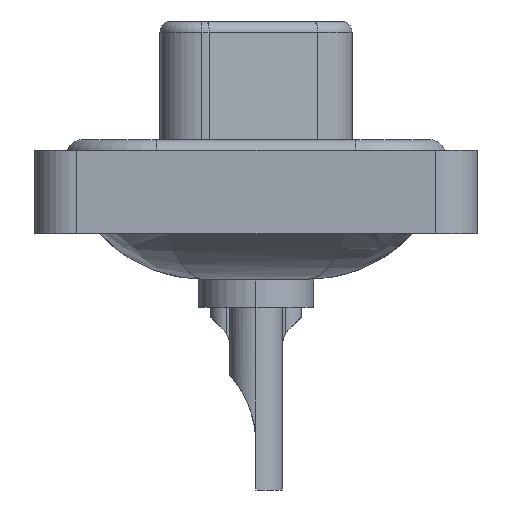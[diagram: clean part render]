
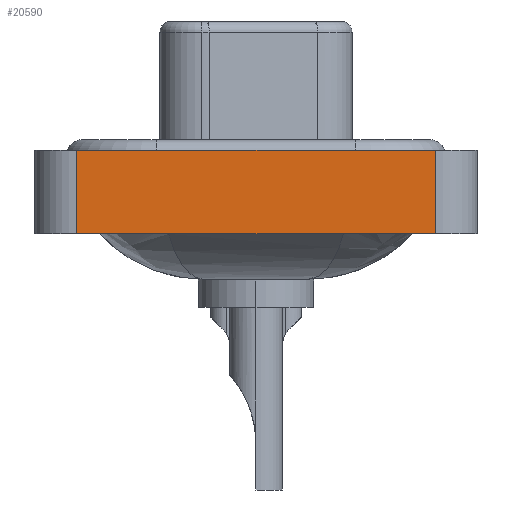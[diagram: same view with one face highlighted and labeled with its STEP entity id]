
A CAD part, left-side view. The second image highlights one B-rep face of the part: STEP entity #20590.
In plain terms, the highlighted planar face has unit normal (-1, 0, 0).
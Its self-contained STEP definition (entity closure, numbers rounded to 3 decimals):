
#236 = ORIENTED_EDGE ( 'NONE', *, *, #13467, .F. ) ;
#2484 = DIRECTION ( 'NONE',  ( 0., 0., 1. ) ) ;
#3083 = FACE_OUTER_BOUND ( 'NONE', #12416, .T. ) ;
#3093 = DIRECTION ( 'NONE',  ( 0., 0., 1. ) ) ;
#3206 = CARTESIAN_POINT ( 'NONE',  ( -7.35, 8.55, -3.6 ) ) ;
#3216 = ORIENTED_EDGE ( 'NONE', *, *, #18373, .T. ) ;
#3691 = AXIS2_PLACEMENT_3D ( 'NONE', #9576, #16239, #12870 ) ;
#4490 = LINE ( 'NONE', #17212, #16554 ) ;
#4629 = VECTOR ( 'NONE', #10904, 1000. ) ;
#5067 = VERTEX_POINT ( 'NONE', #20073 ) ;
#5193 = ORIENTED_EDGE ( 'NONE', *, *, #20450, .F. ) ;
#5450 = VECTOR ( 'NONE', #3093, 1000. ) ;
#5786 = LINE ( 'NONE', #7679, #10081 ) ;
#6405 = CARTESIAN_POINT ( 'NONE',  ( -7.35, -8.55, 0.4 ) ) ;
#6598 = VERTEX_POINT ( 'NONE', #8082 ) ;
#7659 = DIRECTION ( 'NONE',  ( 0., -1., 0. ) ) ;
#7679 = CARTESIAN_POINT ( 'NONE',  ( -7.35, -8.55, -3.6 ) ) ;
#8082 = CARTESIAN_POINT ( 'NONE',  ( -7.35, -8.55, -3.6 ) ) ;
#9355 = PLANE ( 'NONE',  #3691 ) ;
#9576 = CARTESIAN_POINT ( 'NONE',  ( -7.35, -8.55, -3.6 ) ) ;
#10081 = VECTOR ( 'NONE', #2484, 1000. ) ;
#10904 = DIRECTION ( 'NONE',  ( 0., -1., 0. ) ) ;
#12416 = EDGE_LOOP ( 'NONE', ( #19636, #5193, #236, #3216 ) ) ;
#12870 = DIRECTION ( 'NONE',  ( 0., 0., 1. ) ) ;
#13467 = EDGE_CURVE ( 'NONE', #20142, #5067, #15825, .T. ) ;
#13981 = CARTESIAN_POINT ( 'NONE',  ( -7.35, -8.55, -3.6 ) ) ;
#15825 = LINE ( 'NONE', #3206, #5450 ) ;
#16239 = DIRECTION ( 'NONE',  ( -1., 0., 0. ) ) ;
#16554 = VECTOR ( 'NONE', #7659, 1000. ) ;
#17212 = CARTESIAN_POINT ( 'NONE',  ( -7.35, -8.55, 0.4 ) ) ;
#17869 = CARTESIAN_POINT ( 'NONE',  ( -7.35, 8.55, -3.6 ) ) ;
#18373 = EDGE_CURVE ( 'NONE', #20142, #6598, #20451, .T. ) ;
#18743 = EDGE_CURVE ( 'NONE', #6598, #20289, #5786, .T. ) ;
#19636 = ORIENTED_EDGE ( 'NONE', *, *, #18743, .T. ) ;
#20073 = CARTESIAN_POINT ( 'NONE',  ( -7.35, 8.55, 0.4 ) ) ;
#20142 = VERTEX_POINT ( 'NONE', #17869 ) ;
#20289 = VERTEX_POINT ( 'NONE', #6405 ) ;
#20450 = EDGE_CURVE ( 'NONE', #5067, #20289, #4490, .T. ) ;
#20451 = LINE ( 'NONE', #13981, #4629 ) ;
#20590 = ADVANCED_FACE ( 'NONE', ( #3083 ), #9355, .T. ) ;
